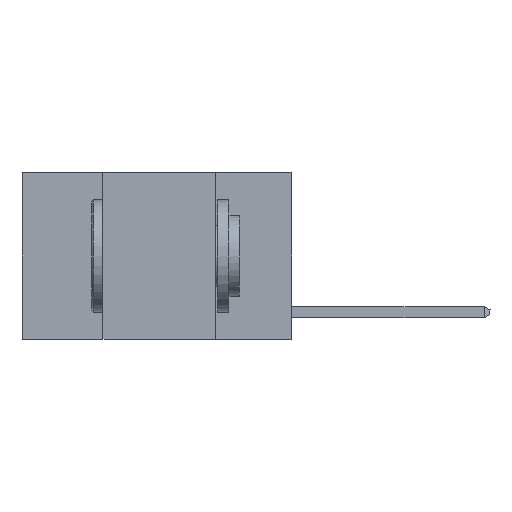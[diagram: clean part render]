
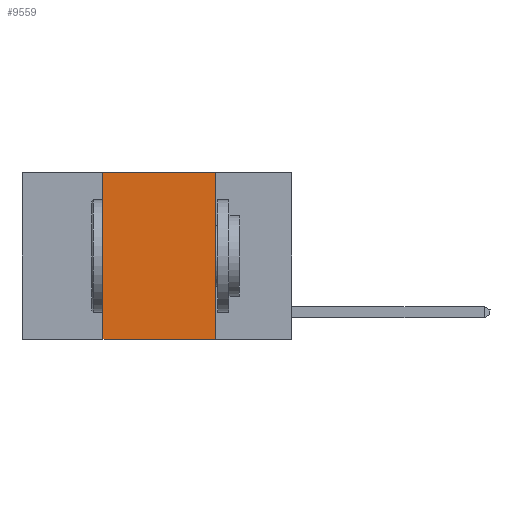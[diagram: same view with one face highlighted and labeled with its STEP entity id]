
A CAD part, left-side view. The second image highlights one B-rep face of the part: STEP entity #9559.
In plain terms, the highlighted planar face has unit normal (-1, 0, 0).
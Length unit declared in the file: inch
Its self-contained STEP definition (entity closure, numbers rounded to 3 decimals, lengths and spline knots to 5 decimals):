
#163 = DIRECTION ( 'NONE',  ( 0., -1., 0. ) ) ;
#295 = EDGE_LOOP ( 'NONE', ( #8917, #7454, #11006, #23124 ) ) ;
#1044 = EDGE_CURVE ( 'NONE', #18137, #18581, #17580, .T. ) ;
#2795 = VECTOR ( 'NONE', #22196, 39.37008 ) ;
#3225 = DIRECTION ( 'NONE',  ( 1., 0., 0. ) ) ;
#3562 = CARTESIAN_POINT ( 'NONE',  ( 0., 0.17, 0. ) ) ;
#3993 = AXIS2_PLACEMENT_3D ( 'NONE', #14314, #3225, #16182 ) ;
#4308 = VECTOR ( 'NONE', #16472, 39.37008 ) ;
#5721 = CARTESIAN_POINT ( 'NONE',  ( 0., 0.6, -0.37 ) ) ;
#7454 = ORIENTED_EDGE ( 'NONE', *, *, #1044, .F. ) ;
#8872 = CARTESIAN_POINT ( 'NONE',  ( 0., 0.17, -0.37 ) ) ;
#8917 = ORIENTED_EDGE ( 'NONE', *, *, #14540, .F. ) ;
#9559 = ADVANCED_FACE ( 'NONE', ( #15163 ), #12490, .F. ) ;
#9675 = CARTESIAN_POINT ( 'NONE',  ( 0., 0.42, 0. ) ) ;
#11006 = ORIENTED_EDGE ( 'NONE', *, *, #19963, .F. ) ;
#12490 = PLANE ( 'NONE',  #3993 ) ;
#12992 = LINE ( 'NONE', #14240, #22215 ) ;
#13344 = VECTOR ( 'NONE', #163, 39.37008 ) ;
#13971 = CARTESIAN_POINT ( 'NONE',  ( 0., 0.42, -0.37 ) ) ;
#14240 = CARTESIAN_POINT ( 'NONE',  ( 0., 0.17, 0. ) ) ;
#14314 = CARTESIAN_POINT ( 'NONE',  ( 0., 0.6, 0. ) ) ;
#14540 = EDGE_CURVE ( 'NONE', #18581, #23145, #12992, .T. ) ;
#15117 = VERTEX_POINT ( 'NONE', #13971 ) ;
#15163 = FACE_OUTER_BOUND ( 'NONE', #295, .T. ) ;
#16182 = DIRECTION ( 'NONE',  ( 0., 0., -1. ) ) ;
#16472 = DIRECTION ( 'NONE',  ( 0., 0., 1. ) ) ;
#17580 = LINE ( 'NONE', #20722, #2795 ) ;
#17678 = LINE ( 'NONE', #5721, #13344 ) ;
#17879 = DIRECTION ( 'NONE',  ( 0., 0., -1. ) ) ;
#18137 = VERTEX_POINT ( 'NONE', #9675 ) ;
#18581 = VERTEX_POINT ( 'NONE', #3562 ) ;
#18708 = EDGE_CURVE ( 'NONE', #15117, #23145, #17678, .T. ) ;
#19072 = LINE ( 'NONE', #20177, #4308 ) ;
#19963 = EDGE_CURVE ( 'NONE', #15117, #18137, #19072, .T. ) ;
#20177 = CARTESIAN_POINT ( 'NONE',  ( 0., 0.42, 0. ) ) ;
#20722 = CARTESIAN_POINT ( 'NONE',  ( 0., 0.6, 0. ) ) ;
#22196 = DIRECTION ( 'NONE',  ( 0., -1., 0. ) ) ;
#22215 = VECTOR ( 'NONE', #17879, 39.37008 ) ;
#23124 = ORIENTED_EDGE ( 'NONE', *, *, #18708, .T. ) ;
#23145 = VERTEX_POINT ( 'NONE', #8872 ) ;
